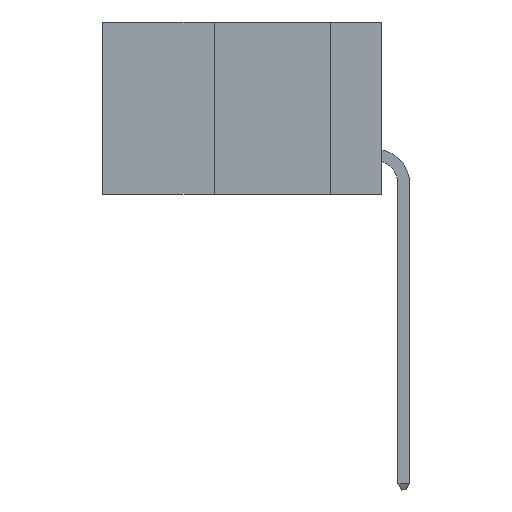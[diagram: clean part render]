
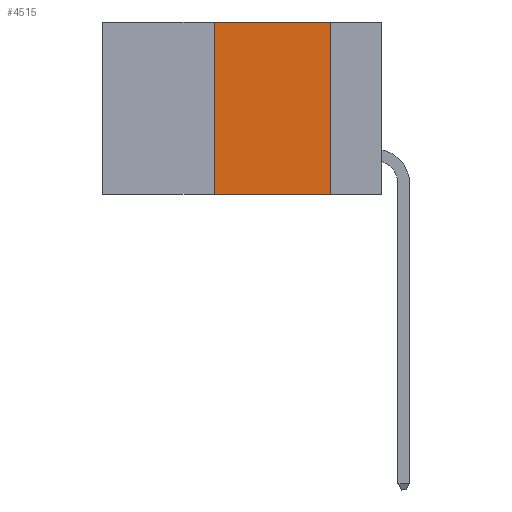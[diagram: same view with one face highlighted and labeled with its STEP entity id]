
A CAD part, left-side view. The second image highlights one B-rep face of the part: STEP entity #4515.
In plain terms, the highlighted planar face has unit normal (-1, 0, 0).
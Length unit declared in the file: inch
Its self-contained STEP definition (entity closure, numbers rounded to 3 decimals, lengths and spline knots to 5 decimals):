
#44 = FACE_OUTER_BOUND ( 'NONE', #23163, .T. ) ;
#1001 = VECTOR ( 'NONE', #13619, 39.37008 ) ;
#1171 = VERTEX_POINT ( 'NONE', #5629 ) ;
#1264 = ORIENTED_EDGE ( 'NONE', *, *, #4647, .F. ) ;
#2373 = VECTOR ( 'NONE', #7734, 39.37008 ) ;
#4250 = LINE ( 'NONE', #23462, #10885 ) ;
#4308 = CARTESIAN_POINT ( 'NONE',  ( 0., 0.11, -0.37 ) ) ;
#4320 = AXIS2_PLACEMENT_3D ( 'NONE', #22058, #18474, #12604 ) ;
#4515 = ADVANCED_FACE ( 'NONE', ( #44 ), #20082, .F. ) ;
#4647 = EDGE_CURVE ( 'NONE', #1171, #5570, #13960, .T. ) ;
#5394 = ORIENTED_EDGE ( 'NONE', *, *, #15753, .T. ) ;
#5570 = VERTEX_POINT ( 'NONE', #12828 ) ;
#5629 = CARTESIAN_POINT ( 'NONE',  ( 0., 0.36, -0.37 ) ) ;
#6965 = LINE ( 'NONE', #17749, #7527 ) ;
#7527 = VECTOR ( 'NONE', #12741, 39.37008 ) ;
#7533 = EDGE_CURVE ( 'NONE', #5570, #21067, #6965, .T. ) ;
#7734 = DIRECTION ( 'NONE',  ( 0., -1., 0. ) ) ;
#9095 = EDGE_CURVE ( 'NONE', #21067, #16261, #4250, .T. ) ;
#9540 = LINE ( 'NONE', #19136, #2373 ) ;
#10885 = VECTOR ( 'NONE', #23384, 39.37008 ) ;
#12604 = DIRECTION ( 'NONE',  ( 0., 0., -1. ) ) ;
#12741 = DIRECTION ( 'NONE',  ( 0., -1., 0. ) ) ;
#12828 = CARTESIAN_POINT ( 'NONE',  ( 0., 0.36, 0. ) ) ;
#13619 = DIRECTION ( 'NONE',  ( 0., 0., 1. ) ) ;
#13949 = CARTESIAN_POINT ( 'NONE',  ( 0., 0.36, 0. ) ) ;
#13960 = LINE ( 'NONE', #13949, #1001 ) ;
#14666 = ORIENTED_EDGE ( 'NONE', *, *, #9095, .F. ) ;
#15227 = ORIENTED_EDGE ( 'NONE', *, *, #7533, .F. ) ;
#15753 = EDGE_CURVE ( 'NONE', #1171, #16261, #9540, .T. ) ;
#16261 = VERTEX_POINT ( 'NONE', #4308 ) ;
#17749 = CARTESIAN_POINT ( 'NONE',  ( 0., 0.6, 0. ) ) ;
#18474 = DIRECTION ( 'NONE',  ( 1., 0., 0. ) ) ;
#18668 = CARTESIAN_POINT ( 'NONE',  ( 0., 0.11, 0. ) ) ;
#19136 = CARTESIAN_POINT ( 'NONE',  ( 0., 0.6, -0.37 ) ) ;
#20082 = PLANE ( 'NONE',  #4320 ) ;
#21067 = VERTEX_POINT ( 'NONE', #18668 ) ;
#22058 = CARTESIAN_POINT ( 'NONE',  ( 0., 0.6, 0. ) ) ;
#23163 = EDGE_LOOP ( 'NONE', ( #14666, #15227, #1264, #5394 ) ) ;
#23384 = DIRECTION ( 'NONE',  ( 0., 0., -1. ) ) ;
#23462 = CARTESIAN_POINT ( 'NONE',  ( 0., 0.11, 0. ) ) ;
